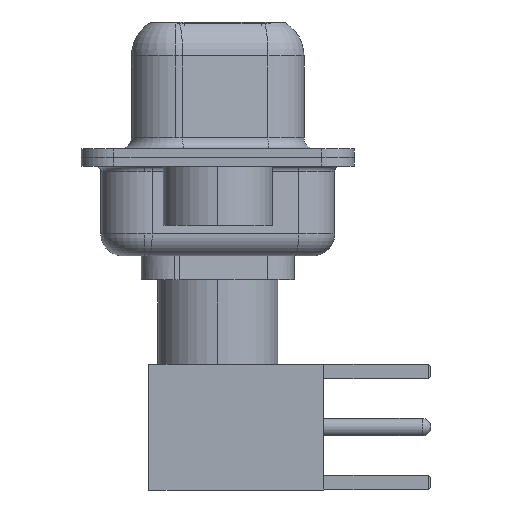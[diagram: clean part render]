
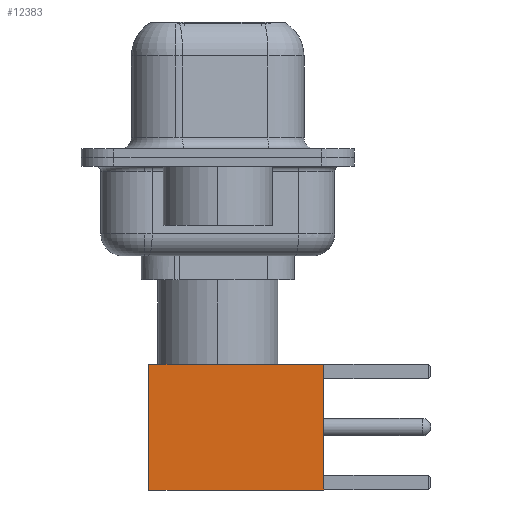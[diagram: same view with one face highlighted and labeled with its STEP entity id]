
A CAD part, left-side view. The second image highlights one B-rep face of the part: STEP entity #12383.
In plain terms, the highlighted face is planar.
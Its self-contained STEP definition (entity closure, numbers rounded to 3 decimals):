
#255 = FACE_OUTER_BOUND ( 'NONE', #9183, .T. ) ;
#1529 = DIRECTION ( 'NONE',  ( 0., 0., -1. ) ) ;
#1634 = DIRECTION ( 'NONE',  ( -1., 0., 0. ) ) ;
#2148 = ORIENTED_EDGE ( 'NONE', *, *, #12868, .T. ) ;
#2566 = LINE ( 'NONE', #8250, #17909 ) ;
#2752 = VECTOR ( 'NONE', #1529, 1000. ) ;
#3402 = CARTESIAN_POINT ( 'NONE',  ( -2.875, 2.875, 0. ) ) ;
#3656 = VECTOR ( 'NONE', #1634, 1000. ) ;
#3952 = AXIS2_PLACEMENT_3D ( 'NONE', #4451, #14422, #17412 ) ;
#4312 = CARTESIAN_POINT ( 'NONE',  ( 2.875, 2.875, 8. ) ) ;
#4451 = CARTESIAN_POINT ( 'NONE',  ( 2.875, 2.875, 0. ) ) ;
#4611 = LINE ( 'NONE', #14394, #3656 ) ;
#5023 = DIRECTION ( 'NONE',  ( -1., 0., 0. ) ) ;
#6728 = CARTESIAN_POINT ( 'NONE',  ( 2.875, 2.875, 0. ) ) ;
#8250 = CARTESIAN_POINT ( 'NONE',  ( -2.875, 2.875, 0. ) ) ;
#9116 = LINE ( 'NONE', #14808, #15790 ) ;
#9183 = EDGE_LOOP ( 'NONE', ( #2148, #11245, #16511, #17870 ) ) ;
#10600 = EDGE_CURVE ( 'NONE', #13558, #18408, #9116, .T. ) ;
#11112 = CARTESIAN_POINT ( 'NONE',  ( -2.875, 2.875, 8. ) ) ;
#11245 = ORIENTED_EDGE ( 'NONE', *, *, #10600, .T. ) ;
#11338 = EDGE_CURVE ( 'NONE', #17233, #18408, #2566, .T. ) ;
#12383 = ADVANCED_FACE ( 'NONE', ( #255 ), #14697, .T. ) ;
#12764 = EDGE_CURVE ( 'NONE', #13201, #17233, #4611, .T. ) ;
#12868 = EDGE_CURVE ( 'NONE', #13201, #13558, #13075, .T. ) ;
#13075 = LINE ( 'NONE', #14301, #2752 ) ;
#13201 = VERTEX_POINT ( 'NONE', #4312 ) ;
#13558 = VERTEX_POINT ( 'NONE', #6728 ) ;
#14301 = CARTESIAN_POINT ( 'NONE',  ( 2.875, 2.875, 0. ) ) ;
#14394 = CARTESIAN_POINT ( 'NONE',  ( 0., 2.875, 8. ) ) ;
#14422 = DIRECTION ( 'NONE',  ( 0., 1., 0. ) ) ;
#14697 = PLANE ( 'NONE',  #3952 ) ;
#14808 = CARTESIAN_POINT ( 'NONE',  ( 0., 2.875, 0. ) ) ;
#15790 = VECTOR ( 'NONE', #5023, 1000. ) ;
#16511 = ORIENTED_EDGE ( 'NONE', *, *, #11338, .F. ) ;
#17233 = VERTEX_POINT ( 'NONE', #11112 ) ;
#17412 = DIRECTION ( 'NONE',  ( 0., 0., 1. ) ) ;
#17870 = ORIENTED_EDGE ( 'NONE', *, *, #12764, .F. ) ;
#17909 = VECTOR ( 'NONE', #18320, 1000. ) ;
#18320 = DIRECTION ( 'NONE',  ( 0., 0., -1. ) ) ;
#18408 = VERTEX_POINT ( 'NONE', #3402 ) ;
